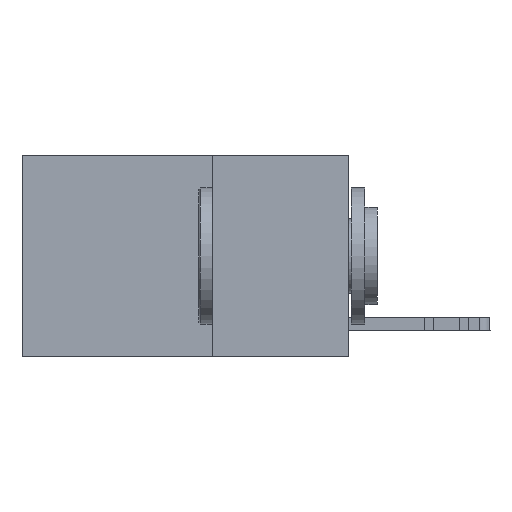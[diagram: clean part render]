
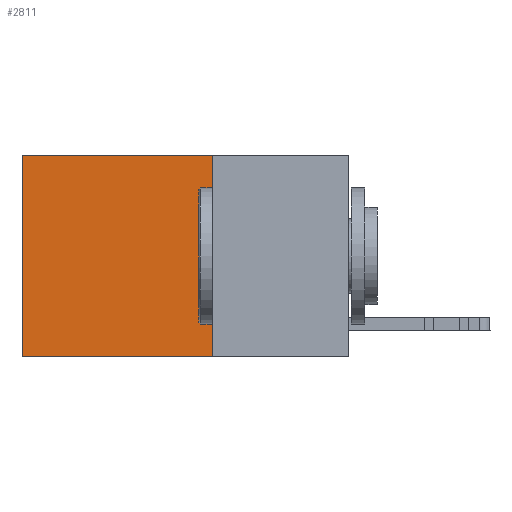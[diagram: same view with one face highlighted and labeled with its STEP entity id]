
A CAD part, left-side view. The second image highlights one B-rep face of the part: STEP entity #2811.
In plain terms, the highlighted planar face has unit normal (-1, 0, 0).
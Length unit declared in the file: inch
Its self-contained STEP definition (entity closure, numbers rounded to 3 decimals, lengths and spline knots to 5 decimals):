
#2057 = CARTESIAN_POINT ( 'NONE',  ( 0.2625, 0.6, -0.37 ) ) ;
#2273 = CARTESIAN_POINT ( 'NONE',  ( 0.2625, 0.25, -0.37 ) ) ;
#2811 = ADVANCED_FACE ( 'NONE', ( #19557 ), #28333, .F. ) ;
#3817 = LINE ( 'NONE', #8074, #13111 ) ;
#4763 = DIRECTION ( 'NONE',  ( 0., 0., -1. ) ) ;
#5665 = CARTESIAN_POINT ( 'NONE',  ( 0.2625, 0.6, 0. ) ) ;
#6575 = EDGE_LOOP ( 'NONE', ( #20549, #9581, #8669, #19767 ) ) ;
#7046 = LINE ( 'NONE', #16247, #20209 ) ;
#7570 = DIRECTION ( 'NONE',  ( 1., 0., 0. ) ) ;
#8074 = CARTESIAN_POINT ( 'NONE',  ( 0.2625, 0.6, 0. ) ) ;
#8669 = ORIENTED_EDGE ( 'NONE', *, *, #8849, .F. ) ;
#8849 = EDGE_CURVE ( 'NONE', #9036, #18589, #7046, .T. ) ;
#9036 = VERTEX_POINT ( 'NONE', #10441 ) ;
#9581 = ORIENTED_EDGE ( 'NONE', *, *, #16718, .F. ) ;
#10441 = CARTESIAN_POINT ( 'NONE',  ( 0.2625, 0.25, 0. ) ) ;
#11548 = CARTESIAN_POINT ( 'NONE',  ( 0.2625, 0.25, -0.37 ) ) ;
#13111 = VECTOR ( 'NONE', #24322, 39.37008 ) ;
#13120 = CARTESIAN_POINT ( 'NONE',  ( 0.2625, 0.25, 0. ) ) ;
#13374 = DIRECTION ( 'NONE',  ( 0., 1., 0. ) ) ;
#16247 = CARTESIAN_POINT ( 'NONE',  ( 0.2625, 0.25, 0. ) ) ;
#16513 = CARTESIAN_POINT ( 'NONE',  ( 0.2625, 0.25, 0. ) ) ;
#16718 = EDGE_CURVE ( 'NONE', #18589, #28806, #29644, .T. ) ;
#17091 = DIRECTION ( 'NONE',  ( 0., 0., -1. ) ) ;
#17151 = EDGE_CURVE ( 'NONE', #20648, #28806, #3817, .T. ) ;
#18589 = VERTEX_POINT ( 'NONE', #2273 ) ;
#19557 = FACE_OUTER_BOUND ( 'NONE', #6575, .T. ) ;
#19767 = ORIENTED_EDGE ( 'NONE', *, *, #28767, .T. ) ;
#20012 = LINE ( 'NONE', #13120, #28572 ) ;
#20209 = VECTOR ( 'NONE', #4763, 39.37008 ) ;
#20549 = ORIENTED_EDGE ( 'NONE', *, *, #17151, .T. ) ;
#20648 = VERTEX_POINT ( 'NONE', #5665 ) ;
#22736 = DIRECTION ( 'NONE',  ( 0., 1., 0. ) ) ;
#24279 = VECTOR ( 'NONE', #13374, 39.37008 ) ;
#24322 = DIRECTION ( 'NONE',  ( 0., 0., -1. ) ) ;
#27961 = AXIS2_PLACEMENT_3D ( 'NONE', #16513, #7570, #17091 ) ;
#28333 = PLANE ( 'NONE',  #27961 ) ;
#28572 = VECTOR ( 'NONE', #22736, 39.37008 ) ;
#28767 = EDGE_CURVE ( 'NONE', #9036, #20648, #20012, .T. ) ;
#28806 = VERTEX_POINT ( 'NONE', #2057 ) ;
#29644 = LINE ( 'NONE', #11548, #24279 ) ;
